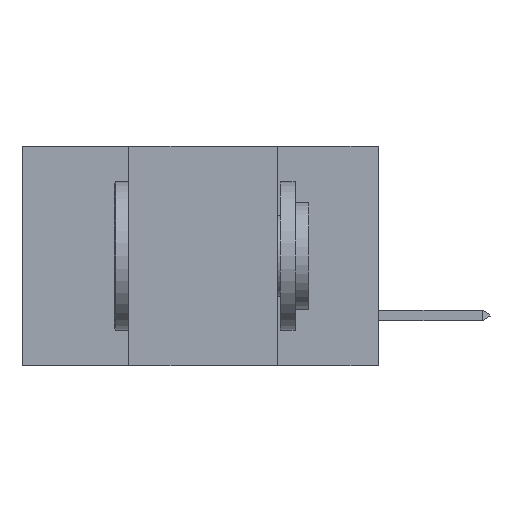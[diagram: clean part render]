
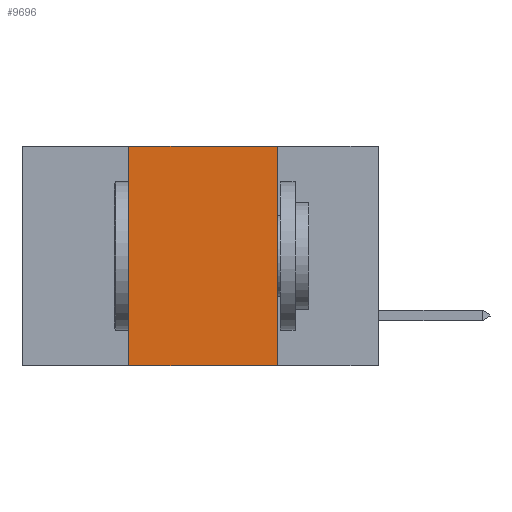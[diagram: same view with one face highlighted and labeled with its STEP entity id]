
A CAD part, left-side view. The second image highlights one B-rep face of the part: STEP entity #9696.
In plain terms, the highlighted planar face has unit normal (-1, 0, 0).
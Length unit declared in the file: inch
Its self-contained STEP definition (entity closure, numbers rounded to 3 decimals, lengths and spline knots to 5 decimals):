
#201 = EDGE_CURVE ( 'NONE', #1384, #11344, #10315, .T. ) ;
#352 = CARTESIAN_POINT ( 'NONE',  ( 0., 0.42, 0. ) ) ;
#622 = LINE ( 'NONE', #12151, #8797 ) ;
#951 = VECTOR ( 'NONE', #5997, 39.37008 ) ;
#960 = EDGE_CURVE ( 'NONE', #12007, #8265, #3130, .T. ) ;
#1116 = DIRECTION ( 'NONE',  ( 0., -1., 0. ) ) ;
#1384 = VERTEX_POINT ( 'NONE', #352 ) ;
#3130 = LINE ( 'NONE', #4212, #13391 ) ;
#3400 = EDGE_CURVE ( 'NONE', #11344, #8265, #4761, .T. ) ;
#3853 = DIRECTION ( 'NONE',  ( 0., -1., 0. ) ) ;
#3871 = CARTESIAN_POINT ( 'NONE',  ( 0., 0.17, 0. ) ) ;
#3947 = FACE_OUTER_BOUND ( 'NONE', #7892, .T. ) ;
#4212 = CARTESIAN_POINT ( 'NONE',  ( 0., 0.6, -0.37 ) ) ;
#4761 = LINE ( 'NONE', #3871, #951 ) ;
#5983 = VECTOR ( 'NONE', #3853, 39.37008 ) ;
#5997 = DIRECTION ( 'NONE',  ( 0., 0., -1. ) ) ;
#6306 = ORIENTED_EDGE ( 'NONE', *, *, #3400, .F. ) ;
#7735 = DIRECTION ( 'NONE',  ( 0., 0., 1. ) ) ;
#7892 = EDGE_LOOP ( 'NONE', ( #6306, #12626, #12312, #9131 ) ) ;
#8233 = CARTESIAN_POINT ( 'NONE',  ( 0., 0.17, 0. ) ) ;
#8265 = VERTEX_POINT ( 'NONE', #10014 ) ;
#8797 = VECTOR ( 'NONE', #7735, 39.37008 ) ;
#8940 = EDGE_CURVE ( 'NONE', #12007, #1384, #622, .T. ) ;
#9131 = ORIENTED_EDGE ( 'NONE', *, *, #960, .T. ) ;
#9696 = ADVANCED_FACE ( 'NONE', ( #3947 ), #11381, .F. ) ;
#10014 = CARTESIAN_POINT ( 'NONE',  ( 0., 0.17, -0.37 ) ) ;
#10315 = LINE ( 'NONE', #11216, #5983 ) ;
#10336 = DIRECTION ( 'NONE',  ( 0., 0., -1. ) ) ;
#10623 = AXIS2_PLACEMENT_3D ( 'NONE', #12300, #12474, #10336 ) ;
#11216 = CARTESIAN_POINT ( 'NONE',  ( 0., 0.6, 0. ) ) ;
#11344 = VERTEX_POINT ( 'NONE', #8233 ) ;
#11381 = PLANE ( 'NONE',  #10623 ) ;
#11431 = CARTESIAN_POINT ( 'NONE',  ( 0., 0.42, -0.37 ) ) ;
#12007 = VERTEX_POINT ( 'NONE', #11431 ) ;
#12151 = CARTESIAN_POINT ( 'NONE',  ( 0., 0.42, 0. ) ) ;
#12300 = CARTESIAN_POINT ( 'NONE',  ( 0., 0.6, 0. ) ) ;
#12312 = ORIENTED_EDGE ( 'NONE', *, *, #8940, .F. ) ;
#12474 = DIRECTION ( 'NONE',  ( 1., 0., 0. ) ) ;
#12626 = ORIENTED_EDGE ( 'NONE', *, *, #201, .F. ) ;
#13391 = VECTOR ( 'NONE', #1116, 39.37008 ) ;
